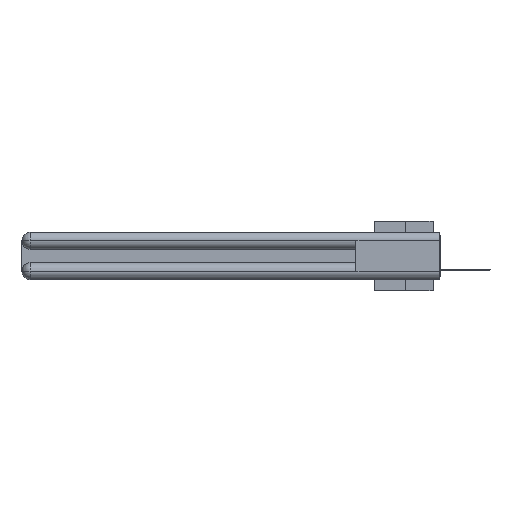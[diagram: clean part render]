
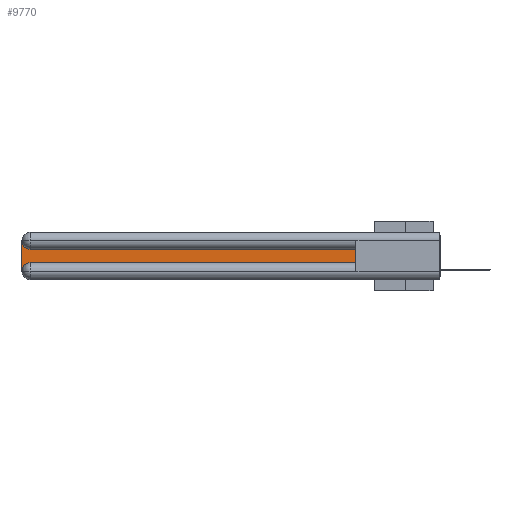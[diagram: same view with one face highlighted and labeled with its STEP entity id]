
A CAD part, left-side view. The second image highlights one B-rep face of the part: STEP entity #9770.
In plain terms, the highlighted planar face has unit normal (-1, 0, 0).
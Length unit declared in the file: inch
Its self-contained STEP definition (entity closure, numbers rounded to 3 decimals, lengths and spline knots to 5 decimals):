
#297 = VERTEX_POINT ( 'NONE', #29202 ) ;
#674 = LINE ( 'NONE', #21799, #19210 ) ;
#1407 = ORIENTED_EDGE ( 'NONE', *, *, #10810, .T. ) ;
#1870 = CARTESIAN_POINT ( 'NONE',  ( 0.075, 2.94, -0.2175 ) ) ;
#2867 = VERTEX_POINT ( 'NONE', #1870 ) ;
#3102 = CARTESIAN_POINT ( 'NONE',  ( 0.075, 3., -0.2775 ) ) ;
#4181 = VECTOR ( 'NONE', #4406, 39.37008 ) ;
#4406 = DIRECTION ( 'NONE',  ( 0., 0., -1. ) ) ;
#5417 = ORIENTED_EDGE ( 'NONE', *, *, #24404, .T. ) ;
#5970 = EDGE_CURVE ( 'NONE', #6550, #25235, #15127, .T. ) ;
#6550 = VERTEX_POINT ( 'NONE', #25619 ) ;
#7842 = FACE_OUTER_BOUND ( 'NONE', #15614, .T. ) ;
#9386 = ORIENTED_EDGE ( 'NONE', *, *, #5970, .T. ) ;
#9770 = ADVANCED_FACE ( 'NONE', ( #7842 ), #16449, .F. ) ;
#9851 = CARTESIAN_POINT ( 'NONE',  ( 0.075, 0.6, -0.1225 ) ) ;
#10125 = ORIENTED_EDGE ( 'NONE', *, *, #26325, .T. ) ;
#10179 = CARTESIAN_POINT ( 'NONE',  ( 0.075, 2.94, -0.2775 ) ) ;
#10277 = LINE ( 'NONE', #33543, #37810 ) ;
#10301 = DIRECTION ( 'NONE',  ( 1., 0., 0. ) ) ;
#10810 = EDGE_CURVE ( 'NONE', #14774, #297, #674, .T. ) ;
#12838 = DIRECTION ( 'NONE',  ( 0., -1., 0. ) ) ;
#13370 = CARTESIAN_POINT ( 'NONE',  ( 0.075, 3., -0.1225 ) ) ;
#13572 = CARTESIAN_POINT ( 'NONE',  ( 0.075, 3., -0.2175 ) ) ;
#14774 = VERTEX_POINT ( 'NONE', #35763 ) ;
#15030 = CARTESIAN_POINT ( 'NONE',  ( 0.075, 2.94, -0.0625 ) ) ;
#15127 = LINE ( 'NONE', #13572, #4181 ) ;
#15614 = EDGE_LOOP ( 'NONE', ( #28113, #21437, #9386, #5417, #10125, #1407 ) ) ;
#16179 = VERTEX_POINT ( 'NONE', #27311 ) ;
#16319 = DIRECTION ( 'NONE',  ( 0., 0., -1. ) ) ;
#16324 = DIRECTION ( 'NONE',  ( 1., 0., 0. ) ) ;
#16449 = PLANE ( 'NONE',  #34596 ) ;
#16643 = CIRCLE ( 'NONE', #28197, 0.06 ) ;
#18918 = DIRECTION ( 'NONE',  ( 0., 1., 0. ) ) ;
#19210 = VECTOR ( 'NONE', #36789, 39.37008 ) ;
#21437 = ORIENTED_EDGE ( 'NONE', *, *, #30371, .T. ) ;
#21518 = LINE ( 'NONE', #9851, #32422 ) ;
#21711 = EDGE_CURVE ( 'NONE', #297, #16179, #21518, .T. ) ;
#21799 = CARTESIAN_POINT ( 'NONE',  ( 0.075, 0.6, -0.2175 ) ) ;
#24404 = EDGE_CURVE ( 'NONE', #25235, #2867, #24637, .T. ) ;
#24637 = CIRCLE ( 'NONE', #37452, 0.06 ) ;
#25235 = VERTEX_POINT ( 'NONE', #3102 ) ;
#25619 = CARTESIAN_POINT ( 'NONE',  ( 0.075, 3., -0.0625 ) ) ;
#26325 = EDGE_CURVE ( 'NONE', #2867, #14774, #10277, .T. ) ;
#27311 = CARTESIAN_POINT ( 'NONE',  ( 0.075, 2.94, -0.1225 ) ) ;
#28113 = ORIENTED_EDGE ( 'NONE', *, *, #21711, .T. ) ;
#28197 = AXIS2_PLACEMENT_3D ( 'NONE', #15030, #35847, #29874 ) ;
#29202 = CARTESIAN_POINT ( 'NONE',  ( 0.075, 0.6, -0.1225 ) ) ;
#29874 = DIRECTION ( 'NONE',  ( 0., 0., -1. ) ) ;
#30371 = EDGE_CURVE ( 'NONE', #16179, #6550, #16643, .T. ) ;
#32422 = VECTOR ( 'NONE', #18918, 39.37008 ) ;
#33543 = CARTESIAN_POINT ( 'NONE',  ( 0.075, 0.6, -0.2175 ) ) ;
#34596 = AXIS2_PLACEMENT_3D ( 'NONE', #13370, #10301, #16319 ) ;
#35763 = CARTESIAN_POINT ( 'NONE',  ( 0.075, 0.6, -0.2175 ) ) ;
#35847 = DIRECTION ( 'NONE',  ( 1., 0., 0. ) ) ;
#36789 = DIRECTION ( 'NONE',  ( 0., 0., 1. ) ) ;
#37452 = AXIS2_PLACEMENT_3D ( 'NONE', #10179, #16324, #37535 ) ;
#37535 = DIRECTION ( 'NONE',  ( 0., 0., -1. ) ) ;
#37810 = VECTOR ( 'NONE', #12838, 39.37008 ) ;
